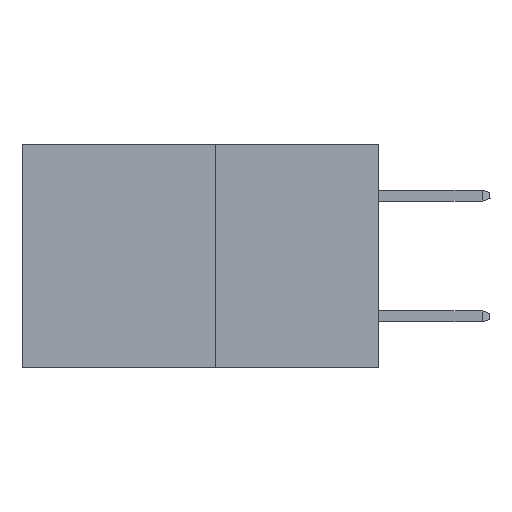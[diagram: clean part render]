
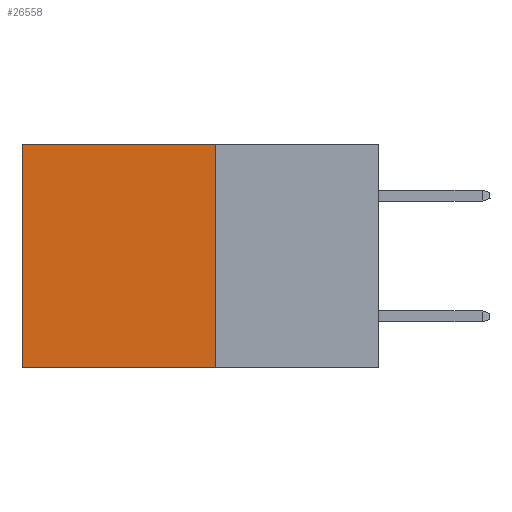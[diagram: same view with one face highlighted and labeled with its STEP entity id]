
A CAD part, left-side view. The second image highlights one B-rep face of the part: STEP entity #26558.
In plain terms, the highlighted planar face has unit normal (-1, 0, 0).
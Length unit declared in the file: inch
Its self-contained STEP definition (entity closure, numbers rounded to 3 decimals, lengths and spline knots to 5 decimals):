
#2222 = FACE_OUTER_BOUND ( 'NONE', #28426, .T. ) ;
#2698 = CARTESIAN_POINT ( 'NONE',  ( 0.277, 0.27, -0.37 ) ) ;
#5072 = LINE ( 'NONE', #26994, #30814 ) ;
#5278 = LINE ( 'NONE', #25175, #31825 ) ;
#5325 = CARTESIAN_POINT ( 'NONE',  ( 0.277, 0.59, -0.37 ) ) ;
#5609 = ORIENTED_EDGE ( 'NONE', *, *, #22299, .T. ) ;
#5747 = VERTEX_POINT ( 'NONE', #7953 ) ;
#6929 = EDGE_CURVE ( 'NONE', #10595, #31044, #21743, .T. ) ;
#7953 = CARTESIAN_POINT ( 'NONE',  ( 0.277, 0.59, 0. ) ) ;
#8191 = EDGE_CURVE ( 'NONE', #5747, #15623, #5072, .T. ) ;
#8563 = LINE ( 'NONE', #20535, #27428 ) ;
#9604 = VECTOR ( 'NONE', #20802, 39.37008 ) ;
#9754 = DIRECTION ( 'NONE',  ( 0., 1., 0. ) ) ;
#10347 = ORIENTED_EDGE ( 'NONE', *, *, #8191, .T. ) ;
#10595 = VERTEX_POINT ( 'NONE', #32698 ) ;
#10765 = CARTESIAN_POINT ( 'NONE',  ( 0.277, 0.27, -0.37 ) ) ;
#13360 = DIRECTION ( 'NONE',  ( 1., 0., 0. ) ) ;
#14222 = DIRECTION ( 'NONE',  ( 0., 0., -1. ) ) ;
#15623 = VERTEX_POINT ( 'NONE', #5325 ) ;
#20535 = CARTESIAN_POINT ( 'NONE',  ( 0.277, 0.27, 0. ) ) ;
#20802 = DIRECTION ( 'NONE',  ( 0., 0., -1. ) ) ;
#21743 = LINE ( 'NONE', #2698, #9604 ) ;
#22299 = EDGE_CURVE ( 'NONE', #10595, #5747, #8563, .T. ) ;
#22873 = EDGE_CURVE ( 'NONE', #31044, #15623, #5278, .T. ) ;
#23099 = DIRECTION ( 'NONE',  ( 0., 1., 0. ) ) ;
#23345 = ORIENTED_EDGE ( 'NONE', *, *, #22873, .F. ) ;
#24769 = CARTESIAN_POINT ( 'NONE',  ( 0.277, 0.27, -0.37 ) ) ;
#25175 = CARTESIAN_POINT ( 'NONE',  ( 0.277, 0.27, -0.37 ) ) ;
#26113 = AXIS2_PLACEMENT_3D ( 'NONE', #10765, #13360, #31285 ) ;
#26149 = PLANE ( 'NONE',  #26113 ) ;
#26558 = ADVANCED_FACE ( 'NONE', ( #2222 ), #26149, .F. ) ;
#26994 = CARTESIAN_POINT ( 'NONE',  ( 0.277, 0.59, -0.37 ) ) ;
#27428 = VECTOR ( 'NONE', #23099, 39.37008 ) ;
#27941 = ORIENTED_EDGE ( 'NONE', *, *, #6929, .F. ) ;
#28426 = EDGE_LOOP ( 'NONE', ( #10347, #23345, #27941, #5609 ) ) ;
#30814 = VECTOR ( 'NONE', #14222, 39.37008 ) ;
#31044 = VERTEX_POINT ( 'NONE', #24769 ) ;
#31285 = DIRECTION ( 'NONE',  ( 0., 0., -1. ) ) ;
#31825 = VECTOR ( 'NONE', #9754, 39.37008 ) ;
#32698 = CARTESIAN_POINT ( 'NONE',  ( 0.277, 0.27, 0. ) ) ;
